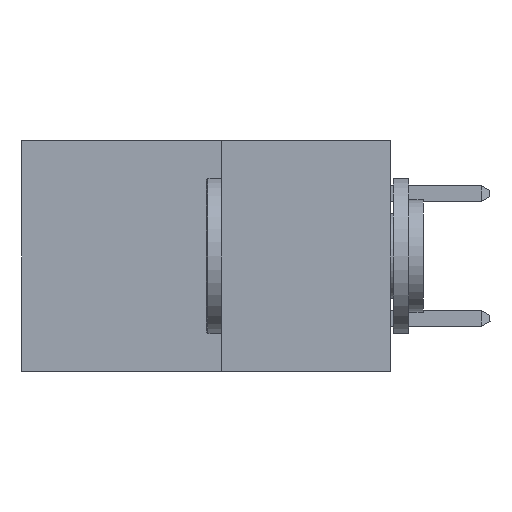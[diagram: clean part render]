
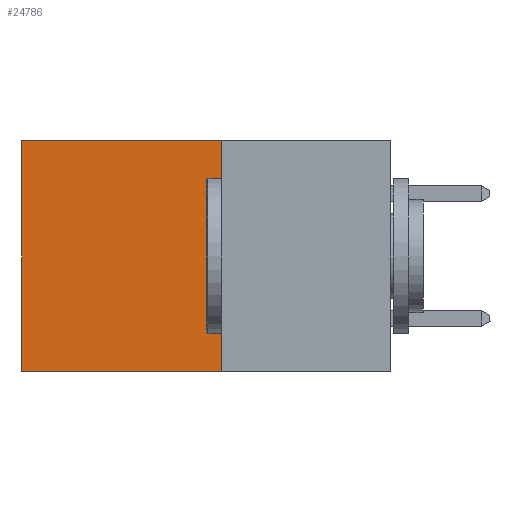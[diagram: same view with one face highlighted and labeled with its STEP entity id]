
A CAD part, left-side view. The second image highlights one B-rep face of the part: STEP entity #24786.
In plain terms, the highlighted planar face has unit normal (-1, 0, 0).
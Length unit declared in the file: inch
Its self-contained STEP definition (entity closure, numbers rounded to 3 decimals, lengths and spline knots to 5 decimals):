
#120 = VERTEX_POINT ( 'NONE', #11084 ) ;
#1395 = AXIS2_PLACEMENT_3D ( 'NONE', #19440, #23427, #11442 ) ;
#2300 = VECTOR ( 'NONE', #6019, 39.37008 ) ;
#2733 = VECTOR ( 'NONE', #24100, 39.37008 ) ;
#3973 = CARTESIAN_POINT ( 'NONE',  ( 0.277, 0.59, -0.37 ) ) ;
#6019 = DIRECTION ( 'NONE',  ( 0., 0., -1. ) ) ;
#6609 = EDGE_CURVE ( 'NONE', #120, #10442, #24140, .T. ) ;
#7670 = DIRECTION ( 'NONE',  ( 0., 0., -1. ) ) ;
#8622 = EDGE_LOOP ( 'NONE', ( #10518, #8704, #16471, #22365 ) ) ;
#8704 = ORIENTED_EDGE ( 'NONE', *, *, #19075, .F. ) ;
#9272 = VECTOR ( 'NONE', #22526, 39.37008 ) ;
#10104 = VERTEX_POINT ( 'NONE', #16465 ) ;
#10442 = VERTEX_POINT ( 'NONE', #11169 ) ;
#10518 = ORIENTED_EDGE ( 'NONE', *, *, #18910, .T. ) ;
#11084 = CARTESIAN_POINT ( 'NONE',  ( 0.277, 0.27, 0. ) ) ;
#11169 = CARTESIAN_POINT ( 'NONE',  ( 0.277, 0.59, 0. ) ) ;
#11442 = DIRECTION ( 'NONE',  ( 0., 0., -1. ) ) ;
#11983 = VECTOR ( 'NONE', #7670, 39.37008 ) ;
#13062 = LINE ( 'NONE', #3973, #2300 ) ;
#14104 = FACE_OUTER_BOUND ( 'NONE', #8622, .T. ) ;
#14936 = CARTESIAN_POINT ( 'NONE',  ( 0.277, 0.27, -0.37 ) ) ;
#16465 = CARTESIAN_POINT ( 'NONE',  ( 0.277, 0.59, -0.37 ) ) ;
#16471 = ORIENTED_EDGE ( 'NONE', *, *, #22202, .F. ) ;
#18595 = CARTESIAN_POINT ( 'NONE',  ( 0.277, 0.27, -0.37 ) ) ;
#18910 = EDGE_CURVE ( 'NONE', #10442, #10104, #13062, .T. ) ;
#19075 = EDGE_CURVE ( 'NONE', #25260, #10104, #19957, .T. ) ;
#19440 = CARTESIAN_POINT ( 'NONE',  ( 0.277, 0.27, -0.37 ) ) ;
#19957 = LINE ( 'NONE', #18595, #9272 ) ;
#21400 = LINE ( 'NONE', #23731, #11983 ) ;
#21447 = PLANE ( 'NONE',  #1395 ) ;
#22202 = EDGE_CURVE ( 'NONE', #120, #25260, #21400, .T. ) ;
#22365 = ORIENTED_EDGE ( 'NONE', *, *, #6609, .T. ) ;
#22526 = DIRECTION ( 'NONE',  ( 0., 1., 0. ) ) ;
#23427 = DIRECTION ( 'NONE',  ( 1., 0., 0. ) ) ;
#23731 = CARTESIAN_POINT ( 'NONE',  ( 0.277, 0.27, -0.37 ) ) ;
#24100 = DIRECTION ( 'NONE',  ( 0., 1., 0. ) ) ;
#24140 = LINE ( 'NONE', #24156, #2733 ) ;
#24156 = CARTESIAN_POINT ( 'NONE',  ( 0.277, 0.27, 0. ) ) ;
#24786 = ADVANCED_FACE ( 'NONE', ( #14104 ), #21447, .F. ) ;
#25260 = VERTEX_POINT ( 'NONE', #14936 ) ;
